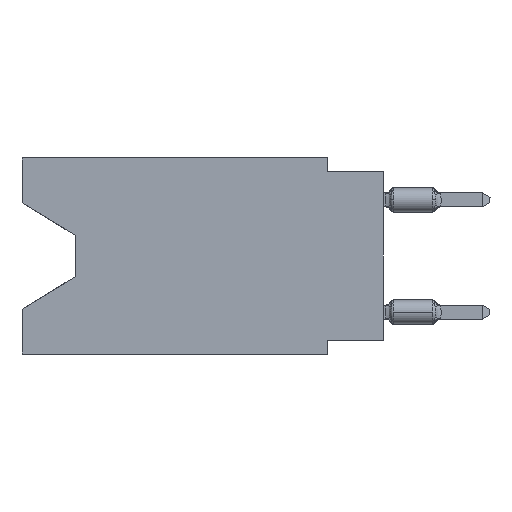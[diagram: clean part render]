
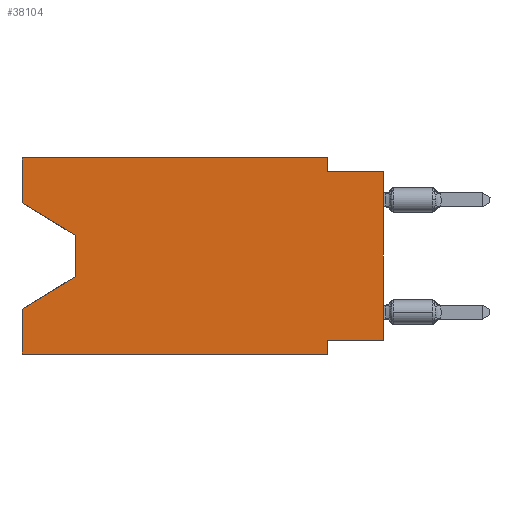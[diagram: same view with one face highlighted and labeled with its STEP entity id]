
A CAD part, left-side view. The second image highlights one B-rep face of the part: STEP entity #38104.
In plain terms, the highlighted planar face has unit normal (-1, 0, 0).
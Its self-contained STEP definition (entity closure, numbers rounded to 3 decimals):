
#59 = VECTOR ( 'NONE', #20295, 1000. ) ;
#1081 = VERTEX_POINT ( 'NONE', #3284 ) ;
#1221 = EDGE_CURVE ( 'NONE', #1081, #2897, #31853, .T. ) ;
#2410 = PLANE ( 'NONE',  #21925 ) ;
#2897 = VERTEX_POINT ( 'NONE', #17642 ) ;
#3200 = LINE ( 'NONE', #6398, #16707 ) ;
#3284 = CARTESIAN_POINT ( 'NONE',  ( 0., 2.54, -0.635 ) ) ;
#3293 = LINE ( 'NONE', #10108, #39367 ) ;
#3331 = LINE ( 'NONE', #25065, #8065 ) ;
#4277 = CARTESIAN_POINT ( 'NONE',  ( 0., 0., -0.635 ) ) ;
#4295 = VECTOR ( 'NONE', #16756, 1000. ) ;
#4723 = VECTOR ( 'NONE', #7003, 1000. ) ;
#4910 = LINE ( 'NONE', #17006, #10486 ) ;
#5072 = LINE ( 'NONE', #17563, #34764 ) ;
#5304 = DIRECTION ( 'NONE',  ( 0., 0., -1. ) ) ;
#5411 = FACE_OUTER_BOUND ( 'NONE', #7112, .T. ) ;
#5415 = CARTESIAN_POINT ( 'NONE',  ( 0., 0., -8.255 ) ) ;
#6398 = CARTESIAN_POINT ( 'NONE',  ( 0., 16.383, 0. ) ) ;
#6431 = CARTESIAN_POINT ( 'NONE',  ( 0., 2.54, -8.89 ) ) ;
#6516 = CARTESIAN_POINT ( 'NONE',  ( 0., 2.54, -8.255 ) ) ;
#6587 = DIRECTION ( 'NONE',  ( 0., 0., 1. ) ) ;
#7003 = DIRECTION ( 'NONE',  ( 0., 0., 1. ) ) ;
#7112 = EDGE_LOOP ( 'NONE', ( #13714, #23195, #29002, #15537, #29744, #12027, #18760, #22252, #17369, #26388, #28129, #9004 ) ) ;
#7876 = EDGE_CURVE ( 'NONE', #7997, #29691, #35602, .T. ) ;
#7997 = VERTEX_POINT ( 'NONE', #19002 ) ;
#8065 = VECTOR ( 'NONE', #37163, 1000. ) ;
#8406 = CARTESIAN_POINT ( 'NONE',  ( 0., 16.383, 0. ) ) ;
#9004 = ORIENTED_EDGE ( 'NONE', *, *, #36230, .F. ) ;
#9550 = VECTOR ( 'NONE', #39238, 1000. ) ;
#10108 = CARTESIAN_POINT ( 'NONE',  ( 0., 2.54, -8.89 ) ) ;
#10486 = VECTOR ( 'NONE', #29283, 1000. ) ;
#10645 = VECTOR ( 'NONE', #28427, 1000. ) ;
#11801 = EDGE_CURVE ( 'NONE', #13591, #24702, #34806, .T. ) ;
#11848 = DIRECTION ( 'NONE',  ( 1., 0., 0. ) ) ;
#12017 = LINE ( 'NONE', #26544, #9550 ) ;
#12027 = ORIENTED_EDGE ( 'NONE', *, *, #39055, .F. ) ;
#12164 = DIRECTION ( 'NONE',  ( 0., -0.855, -0.519 ) ) ;
#12437 = CARTESIAN_POINT ( 'NONE',  ( 0., 16.383, 0. ) ) ;
#13591 = VERTEX_POINT ( 'NONE', #33322 ) ;
#13627 = EDGE_CURVE ( 'NONE', #14182, #31088, #15953, .T. ) ;
#13714 = ORIENTED_EDGE ( 'NONE', *, *, #14346, .T. ) ;
#14182 = VERTEX_POINT ( 'NONE', #5415 ) ;
#14346 = EDGE_CURVE ( 'NONE', #18036, #19959, #15079, .T. ) ;
#15079 = LINE ( 'NONE', #30572, #38346 ) ;
#15537 = ORIENTED_EDGE ( 'NONE', *, *, #11801, .F. ) ;
#15953 = LINE ( 'NONE', #28233, #10645 ) ;
#16199 = CARTESIAN_POINT ( 'NONE',  ( 0., 16.383, -6.852 ) ) ;
#16707 = VECTOR ( 'NONE', #6587, 1000. ) ;
#16756 = DIRECTION ( 'NONE',  ( 0., -1., 0. ) ) ;
#17006 = CARTESIAN_POINT ( 'NONE',  ( 0., 13.97, -5.385 ) ) ;
#17358 = EDGE_CURVE ( 'NONE', #13591, #26704, #12017, .T. ) ;
#17369 = ORIENTED_EDGE ( 'NONE', *, *, #1221, .F. ) ;
#17563 = CARTESIAN_POINT ( 'NONE',  ( 0., 0., 0. ) ) ;
#17642 = CARTESIAN_POINT ( 'NONE',  ( 0., 0., -0.635 ) ) ;
#18036 = VERTEX_POINT ( 'NONE', #32378 ) ;
#18576 = CARTESIAN_POINT ( 'NONE',  ( 0., 13.97, -5.385 ) ) ;
#18760 = ORIENTED_EDGE ( 'NONE', *, *, #13627, .F. ) ;
#19002 = CARTESIAN_POINT ( 'NONE',  ( 0., 16.383, 0. ) ) ;
#19959 = VERTEX_POINT ( 'NONE', #37362 ) ;
#19988 = EDGE_CURVE ( 'NONE', #29691, #1081, #3331, .T. ) ;
#20295 = DIRECTION ( 'NONE',  ( 0., -1., 0. ) ) ;
#20584 = DIRECTION ( 'NONE',  ( 0., 0., 1. ) ) ;
#21410 = EDGE_CURVE ( 'NONE', #25191, #24702, #4910, .T. ) ;
#21925 = AXIS2_PLACEMENT_3D ( 'NONE', #12437, #11848, #27363 ) ;
#22252 = ORIENTED_EDGE ( 'NONE', *, *, #37242, .T. ) ;
#23195 = ORIENTED_EDGE ( 'NONE', *, *, #29123, .T. ) ;
#23856 = CARTESIAN_POINT ( 'NONE',  ( 0., 2.54, 0. ) ) ;
#24026 = LINE ( 'NONE', #27660, #28102 ) ;
#24702 = VERTEX_POINT ( 'NONE', #16199 ) ;
#25065 = CARTESIAN_POINT ( 'NONE',  ( 0., 2.54, 0. ) ) ;
#25191 = VERTEX_POINT ( 'NONE', #18576 ) ;
#25230 = DIRECTION ( 'NONE',  ( 0., 0., -1. ) ) ;
#26388 = ORIENTED_EDGE ( 'NONE', *, *, #19988, .F. ) ;
#26544 = CARTESIAN_POINT ( 'NONE',  ( 0., 16.383, -8.89 ) ) ;
#26704 = VERTEX_POINT ( 'NONE', #6431 ) ;
#27363 = DIRECTION ( 'NONE',  ( 0., 0., -1. ) ) ;
#27660 = CARTESIAN_POINT ( 'NONE',  ( 0., 13.97, -3.505 ) ) ;
#28102 = VECTOR ( 'NONE', #5304, 1000. ) ;
#28129 = ORIENTED_EDGE ( 'NONE', *, *, #7876, .F. ) ;
#28233 = CARTESIAN_POINT ( 'NONE',  ( 0., 0., -8.255 ) ) ;
#28427 = DIRECTION ( 'NONE',  ( 0., 1., 0. ) ) ;
#29002 = ORIENTED_EDGE ( 'NONE', *, *, #21410, .T. ) ;
#29123 = EDGE_CURVE ( 'NONE', #19959, #25191, #24026, .T. ) ;
#29283 = DIRECTION ( 'NONE',  ( 0., 0.855, -0.519 ) ) ;
#29691 = VERTEX_POINT ( 'NONE', #23856 ) ;
#29744 = ORIENTED_EDGE ( 'NONE', *, *, #17358, .T. ) ;
#30572 = CARTESIAN_POINT ( 'NONE',  ( 0., 16.383, -2.038 ) ) ;
#31088 = VERTEX_POINT ( 'NONE', #6516 ) ;
#31853 = LINE ( 'NONE', #4277, #4295 ) ;
#32378 = CARTESIAN_POINT ( 'NONE',  ( 0., 16.383, -2.038 ) ) ;
#33322 = CARTESIAN_POINT ( 'NONE',  ( 0., 16.383, -8.89 ) ) ;
#34764 = VECTOR ( 'NONE', #20584, 1000. ) ;
#34806 = LINE ( 'NONE', #38028, #4723 ) ;
#35602 = LINE ( 'NONE', #8406, #59 ) ;
#36230 = EDGE_CURVE ( 'NONE', #18036, #7997, #3200, .T. ) ;
#37163 = DIRECTION ( 'NONE',  ( 0., 0., -1. ) ) ;
#37242 = EDGE_CURVE ( 'NONE', #14182, #2897, #5072, .T. ) ;
#37362 = CARTESIAN_POINT ( 'NONE',  ( 0., 13.97, -3.505 ) ) ;
#38028 = CARTESIAN_POINT ( 'NONE',  ( 0., 16.383, 0. ) ) ;
#38104 = ADVANCED_FACE ( 'NONE', ( #5411 ), #2410, .F. ) ;
#38346 = VECTOR ( 'NONE', #12164, 1000. ) ;
#39055 = EDGE_CURVE ( 'NONE', #31088, #26704, #3293, .T. ) ;
#39238 = DIRECTION ( 'NONE',  ( 0., -1., 0. ) ) ;
#39367 = VECTOR ( 'NONE', #25230, 1000. ) ;
